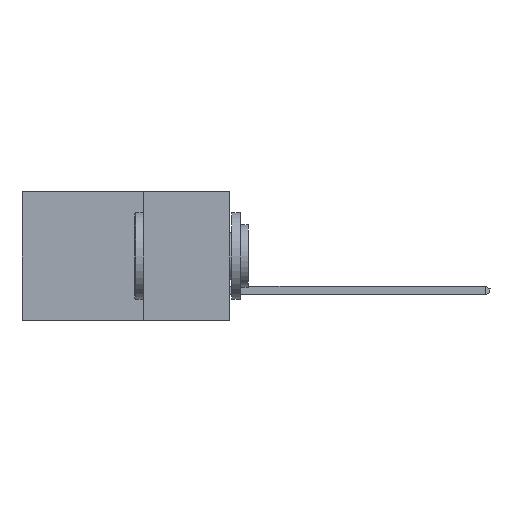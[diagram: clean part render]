
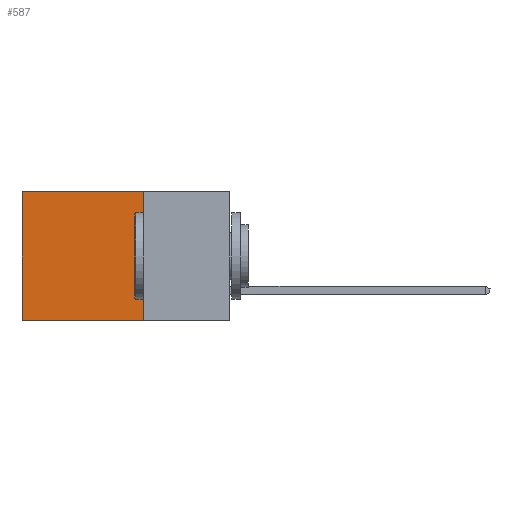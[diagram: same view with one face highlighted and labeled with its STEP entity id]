
A CAD part, left-side view. The second image highlights one B-rep face of the part: STEP entity #587.
In plain terms, the highlighted planar face has unit normal (-1, 0, 0).
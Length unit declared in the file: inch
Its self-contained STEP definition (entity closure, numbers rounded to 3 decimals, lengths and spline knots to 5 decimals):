
#257 = LINE ( 'NONE', #8475, #349 ) ;
#349 = VECTOR ( 'NONE', #2549, 39.37008 ) ;
#416 = DIRECTION ( 'NONE',  ( 0., 1., 0. ) ) ;
#587 = ADVANCED_FACE ( 'NONE', ( #8339 ), #6260, .F. ) ;
#1034 = EDGE_CURVE ( 'NONE', #6479, #1790, #6842, .T. ) ;
#1518 = VECTOR ( 'NONE', #416, 39.37008 ) ;
#1765 = DIRECTION ( 'NONE',  ( 0., 0., -1. ) ) ;
#1790 = VERTEX_POINT ( 'NONE', #5102 ) ;
#1863 = LINE ( 'NONE', #7847, #1518 ) ;
#2463 = ORIENTED_EDGE ( 'NONE', *, *, #4642, .T. ) ;
#2549 = DIRECTION ( 'NONE',  ( 0., 0., -1. ) ) ;
#2585 = AXIS2_PLACEMENT_3D ( 'NONE', #6115, #4577, #1765 ) ;
#2586 = VERTEX_POINT ( 'NONE', #9755 ) ;
#2757 = EDGE_CURVE ( 'NONE', #3732, #2586, #257, .T. ) ;
#2792 = CARTESIAN_POINT ( 'NONE',  ( 0.2615, 0.25, 0. ) ) ;
#3037 = DIRECTION ( 'NONE',  ( 0., 1., 0. ) ) ;
#3732 = VERTEX_POINT ( 'NONE', #9273 ) ;
#4577 = DIRECTION ( 'NONE',  ( 1., 0., 0. ) ) ;
#4642 = EDGE_CURVE ( 'NONE', #6479, #3732, #1863, .T. ) ;
#4720 = DIRECTION ( 'NONE',  ( 0., 0., -1. ) ) ;
#5043 = ORIENTED_EDGE ( 'NONE', *, *, #2757, .T. ) ;
#5102 = CARTESIAN_POINT ( 'NONE',  ( 0.2615, 0.25, -0.37 ) ) ;
#5746 = ORIENTED_EDGE ( 'NONE', *, *, #7327, .F. ) ;
#5799 = ORIENTED_EDGE ( 'NONE', *, *, #1034, .F. ) ;
#6115 = CARTESIAN_POINT ( 'NONE',  ( 0.2615, 0.25, -0.37 ) ) ;
#6260 = PLANE ( 'NONE',  #2585 ) ;
#6399 = VECTOR ( 'NONE', #3037, 39.37008 ) ;
#6479 = VERTEX_POINT ( 'NONE', #2792 ) ;
#6798 = LINE ( 'NONE', #9754, #6399 ) ;
#6805 = VECTOR ( 'NONE', #4720, 39.37008 ) ;
#6842 = LINE ( 'NONE', #7682, #6805 ) ;
#7327 = EDGE_CURVE ( 'NONE', #1790, #2586, #6798, .T. ) ;
#7682 = CARTESIAN_POINT ( 'NONE',  ( 0.2615, 0.25, -0.37 ) ) ;
#7847 = CARTESIAN_POINT ( 'NONE',  ( 0.2615, 0.25, 0. ) ) ;
#8339 = FACE_OUTER_BOUND ( 'NONE', #8654, .T. ) ;
#8475 = CARTESIAN_POINT ( 'NONE',  ( 0.2615, 0.6, -0.37 ) ) ;
#8654 = EDGE_LOOP ( 'NONE', ( #5043, #5746, #5799, #2463 ) ) ;
#9273 = CARTESIAN_POINT ( 'NONE',  ( 0.2615, 0.6, 0. ) ) ;
#9754 = CARTESIAN_POINT ( 'NONE',  ( 0.2615, 0.25, -0.37 ) ) ;
#9755 = CARTESIAN_POINT ( 'NONE',  ( 0.2615, 0.6, -0.37 ) ) ;
